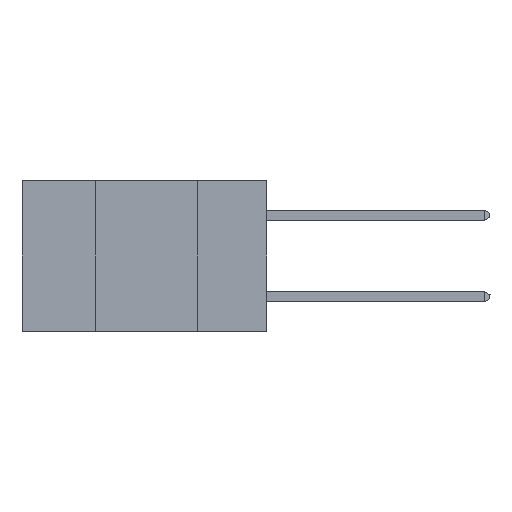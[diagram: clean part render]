
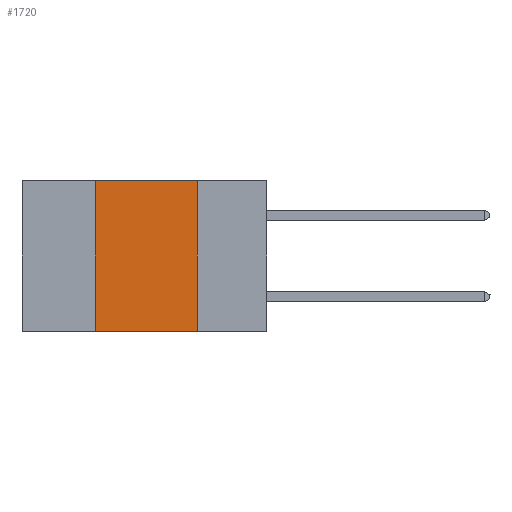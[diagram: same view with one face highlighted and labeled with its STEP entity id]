
A CAD part, left-side view. The second image highlights one B-rep face of the part: STEP entity #1720.
In plain terms, the highlighted planar face has unit normal (-1, 0, 0).
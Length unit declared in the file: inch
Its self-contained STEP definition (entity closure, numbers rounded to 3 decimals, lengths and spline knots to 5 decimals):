
#86 = ORIENTED_EDGE ( 'NONE', *, *, #9848, .F. ) ;
#187 = CARTESIAN_POINT ( 'NONE',  ( 0., 0.42, 0. ) ) ;
#636 = CARTESIAN_POINT ( 'NONE',  ( 0., 0.17, 0. ) ) ;
#1707 = LINE ( 'NONE', #187, #10687 ) ;
#1720 = ADVANCED_FACE ( 'NONE', ( #14334 ), #21356, .F. ) ;
#1970 = VECTOR ( 'NONE', #22467, 39.37008 ) ;
#2615 = CARTESIAN_POINT ( 'NONE',  ( 0., 0.6, 0. ) ) ;
#2771 = DIRECTION ( 'NONE',  ( 0., -1., 0. ) ) ;
#3330 = CARTESIAN_POINT ( 'NONE',  ( 0., 0.6, 0. ) ) ;
#3941 = VERTEX_POINT ( 'NONE', #15389 ) ;
#5150 = DIRECTION ( 'NONE',  ( 1., 0., 0. ) ) ;
#6957 = EDGE_CURVE ( 'NONE', #14154, #10833, #14396, .T. ) ;
#7749 = LINE ( 'NONE', #2615, #13708 ) ;
#8747 = EDGE_CURVE ( 'NONE', #3941, #12331, #7749, .T. ) ;
#8959 = CARTESIAN_POINT ( 'NONE',  ( 0., 0.42, -0.37 ) ) ;
#9848 = EDGE_CURVE ( 'NONE', #12331, #10833, #22283, .T. ) ;
#10272 = ORIENTED_EDGE ( 'NONE', *, *, #6957, .T. ) ;
#10687 = VECTOR ( 'NONE', #21176, 39.37008 ) ;
#10833 = VERTEX_POINT ( 'NONE', #11681 ) ;
#11681 = CARTESIAN_POINT ( 'NONE',  ( 0., 0.17, -0.37 ) ) ;
#12331 = VERTEX_POINT ( 'NONE', #636 ) ;
#12452 = VECTOR ( 'NONE', #18114, 39.37008 ) ;
#13526 = AXIS2_PLACEMENT_3D ( 'NONE', #3330, #5150, #16345 ) ;
#13708 = VECTOR ( 'NONE', #2771, 39.37008 ) ;
#13723 = ORIENTED_EDGE ( 'NONE', *, *, #20285, .F. ) ;
#14154 = VERTEX_POINT ( 'NONE', #8959 ) ;
#14334 = FACE_OUTER_BOUND ( 'NONE', #21603, .T. ) ;
#14396 = LINE ( 'NONE', #16544, #1970 ) ;
#15389 = CARTESIAN_POINT ( 'NONE',  ( 0., 0.42, 0. ) ) ;
#16061 = ORIENTED_EDGE ( 'NONE', *, *, #8747, .F. ) ;
#16345 = DIRECTION ( 'NONE',  ( 0., 0., -1. ) ) ;
#16544 = CARTESIAN_POINT ( 'NONE',  ( 0., 0.6, -0.37 ) ) ;
#18114 = DIRECTION ( 'NONE',  ( 0., 0., -1. ) ) ;
#20285 = EDGE_CURVE ( 'NONE', #14154, #3941, #1707, .T. ) ;
#21176 = DIRECTION ( 'NONE',  ( 0., 0., 1. ) ) ;
#21356 = PLANE ( 'NONE',  #13526 ) ;
#21603 = EDGE_LOOP ( 'NONE', ( #86, #16061, #13723, #10272 ) ) ;
#22283 = LINE ( 'NONE', #23931, #12452 ) ;
#22467 = DIRECTION ( 'NONE',  ( 0., -1., 0. ) ) ;
#23931 = CARTESIAN_POINT ( 'NONE',  ( 0., 0.17, 0. ) ) ;
